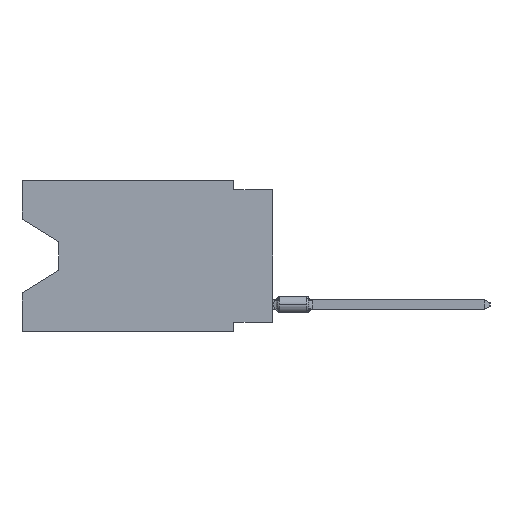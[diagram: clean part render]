
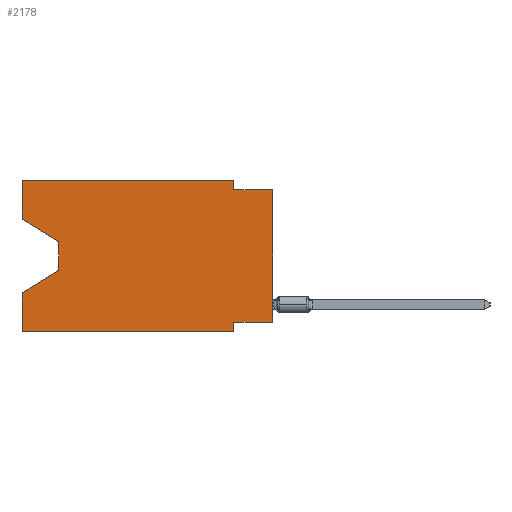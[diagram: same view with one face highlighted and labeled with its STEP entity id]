
A CAD part, left-side view. The second image highlights one B-rep face of the part: STEP entity #2178.
In plain terms, the highlighted planar face has unit normal (-1, 0, 0).
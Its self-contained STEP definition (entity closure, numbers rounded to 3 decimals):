
#2178 = ADVANCED_FACE ( 'NONE', ( #44456 ), #65878, .F. ) ;
#2504 = VERTEX_POINT ( 'NONE', #70240 ) ;
#3340 = ORIENTED_EDGE ( 'NONE', *, *, #38763, .F. ) ;
#3850 = VERTEX_POINT ( 'NONE', #56919 ) ;
#5890 = EDGE_CURVE ( 'NONE', #26819, #31688, #14589, .T. ) ;
#6187 = LINE ( 'NONE', #35373, #51066 ) ;
#7410 = VECTOR ( 'NONE', #53629, 1000. ) ;
#7866 = VECTOR ( 'NONE', #25039, 1000. ) ;
#8179 = EDGE_CURVE ( 'NONE', #27010, #69252, #20210, .T. ) ;
#8800 = DIRECTION ( 'NONE',  ( 0., 0., -1. ) ) ;
#9106 = ORIENTED_EDGE ( 'NONE', *, *, #55734, .T. ) ;
#9294 = CARTESIAN_POINT ( 'NONE',  ( 0., 2.54, 0. ) ) ;
#14589 = LINE ( 'NONE', #32712, #46270 ) ;
#15774 = EDGE_CURVE ( 'NONE', #3850, #2504, #6187, .T. ) ;
#16365 = CARTESIAN_POINT ( 'NONE',  ( 0., 0., -0.635 ) ) ;
#16790 = CARTESIAN_POINT ( 'NONE',  ( 0., 2.54, -0.635 ) ) ;
#17894 = VECTOR ( 'NONE', #57328, 1000. ) ;
#20210 = LINE ( 'NONE', #42770, #64176 ) ;
#23904 = EDGE_CURVE ( 'NONE', #27010, #28588, #71907, .T. ) ;
#24351 = ORIENTED_EDGE ( 'NONE', *, *, #54726, .F. ) ;
#24639 = ORIENTED_EDGE ( 'NONE', *, *, #45463, .F. ) ;
#25039 = DIRECTION ( 'NONE',  ( 0., 0., -1. ) ) ;
#26361 = DIRECTION ( 'NONE',  ( 0., 0., -1. ) ) ;
#26819 = VERTEX_POINT ( 'NONE', #43142 ) ;
#27010 = VERTEX_POINT ( 'NONE', #58485 ) ;
#27949 = DIRECTION ( 'NONE',  ( 0., 0., 1. ) ) ;
#28588 = VERTEX_POINT ( 'NONE', #60197 ) ;
#30990 = EDGE_CURVE ( 'NONE', #57679, #66327, #49240, .T. ) ;
#31113 = LINE ( 'NONE', #32211, #7410 ) ;
#31688 = VERTEX_POINT ( 'NONE', #71348 ) ;
#32211 = CARTESIAN_POINT ( 'NONE',  ( 0., 16.383, 0. ) ) ;
#32712 = CARTESIAN_POINT ( 'NONE',  ( 0., 16.383, -2.546 ) ) ;
#33764 = DIRECTION ( 'NONE',  ( 0., -1., 0. ) ) ;
#34282 = DIRECTION ( 'NONE',  ( 0., 0., 1. ) ) ;
#34669 = ORIENTED_EDGE ( 'NONE', *, *, #5890, .T. ) ;
#35373 = CARTESIAN_POINT ( 'NONE',  ( 0., 0., 0. ) ) ;
#37228 = DIRECTION ( 'NONE',  ( 0., -1., 0. ) ) ;
#37519 = ORIENTED_EDGE ( 'NONE', *, *, #69914, .F. ) ;
#38763 = EDGE_CURVE ( 'NONE', #63058, #69252, #70104, .T. ) ;
#39256 = LINE ( 'NONE', #56597, #60037 ) ;
#39663 = EDGE_CURVE ( 'NONE', #66327, #72418, #45112, .T. ) ;
#40683 = LINE ( 'NONE', #16365, #62429 ) ;
#40953 = ORIENTED_EDGE ( 'NONE', *, *, #30990, .F. ) ;
#41041 = DIRECTION ( 'NONE',  ( 0., 0., -1. ) ) ;
#41968 = CARTESIAN_POINT ( 'NONE',  ( 0., 2.54, -9.906 ) ) ;
#42770 = CARTESIAN_POINT ( 'NONE',  ( 0., 16.383, -9.906 ) ) ;
#43142 = CARTESIAN_POINT ( 'NONE',  ( 0., 16.383, -2.546 ) ) ;
#44456 = FACE_OUTER_BOUND ( 'NONE', #56795, .T. ) ;
#45112 = LINE ( 'NONE', #63183, #51645 ) ;
#45463 = EDGE_CURVE ( 'NONE', #26819, #57679, #31113, .T. ) ;
#45885 = VERTEX_POINT ( 'NONE', #64636 ) ;
#46270 = VECTOR ( 'NONE', #53761, 1000. ) ;
#47268 = VECTOR ( 'NONE', #71763, 1000. ) ;
#47351 = CARTESIAN_POINT ( 'NONE',  ( 0., 13.97, -5.893 ) ) ;
#48974 = CARTESIAN_POINT ( 'NONE',  ( 0., 2.54, -9.271 ) ) ;
#49240 = LINE ( 'NONE', #70301, #47268 ) ;
#49623 = DIRECTION ( 'NONE',  ( 1., 0., 0. ) ) ;
#50493 = ORIENTED_EDGE ( 'NONE', *, *, #39663, .F. ) ;
#50818 = CARTESIAN_POINT ( 'NONE',  ( 0., 16.383, 0. ) ) ;
#51066 = VECTOR ( 'NONE', #34282, 1000. ) ;
#51645 = VECTOR ( 'NONE', #41041, 1000. ) ;
#53629 = DIRECTION ( 'NONE',  ( 0., 0., 1. ) ) ;
#53761 = DIRECTION ( 'NONE',  ( 0., -0.855, -0.519 ) ) ;
#54726 = EDGE_CURVE ( 'NONE', #72418, #2504, #40683, .T. ) ;
#55734 = EDGE_CURVE ( 'NONE', #31688, #45885, #59415, .T. ) ;
#55890 = CARTESIAN_POINT ( 'NONE',  ( 0., 16.383, 0. ) ) ;
#56597 = CARTESIAN_POINT ( 'NONE',  ( 0., 0., -9.271 ) ) ;
#56795 = EDGE_LOOP ( 'NONE', ( #34669, #9106, #67326, #58137, #65698, #3340, #37519, #58535, #24351, #50493, #40953, #24639 ) ) ;
#56919 = CARTESIAN_POINT ( 'NONE',  ( 0., 0., -9.271 ) ) ;
#57328 = DIRECTION ( 'NONE',  ( 0., 0.855, -0.519 ) ) ;
#57679 = VERTEX_POINT ( 'NONE', #50818 ) ;
#58137 = ORIENTED_EDGE ( 'NONE', *, *, #23904, .F. ) ;
#58485 = CARTESIAN_POINT ( 'NONE',  ( 0., 16.383, -9.906 ) ) ;
#58535 = ORIENTED_EDGE ( 'NONE', *, *, #15774, .T. ) ;
#59415 = LINE ( 'NONE', #70140, #62529 ) ;
#60037 = VECTOR ( 'NONE', #62144, 1000. ) ;
#60197 = CARTESIAN_POINT ( 'NONE',  ( 0., 16.383, -7.36 ) ) ;
#62144 = DIRECTION ( 'NONE',  ( 0., 1., 0. ) ) ;
#62429 = VECTOR ( 'NONE', #33764, 1000. ) ;
#62529 = VECTOR ( 'NONE', #8800, 1000. ) ;
#63058 = VERTEX_POINT ( 'NONE', #48974 ) ;
#63183 = CARTESIAN_POINT ( 'NONE',  ( 0., 2.54, 0. ) ) ;
#63957 = LINE ( 'NONE', #47351, #17894 ) ;
#64176 = VECTOR ( 'NONE', #37228, 1000. ) ;
#64636 = CARTESIAN_POINT ( 'NONE',  ( 0., 13.97, -5.893 ) ) ;
#64780 = AXIS2_PLACEMENT_3D ( 'NONE', #55890, #49623, #26361 ) ;
#65698 = ORIENTED_EDGE ( 'NONE', *, *, #8179, .T. ) ;
#65878 = PLANE ( 'NONE',  #64780 ) ;
#66327 = VERTEX_POINT ( 'NONE', #9294 ) ;
#67089 = CARTESIAN_POINT ( 'NONE',  ( 0., 16.383, 0. ) ) ;
#67326 = ORIENTED_EDGE ( 'NONE', *, *, #72991, .T. ) ;
#68078 = VECTOR ( 'NONE', #27949, 1000. ) ;
#69252 = VERTEX_POINT ( 'NONE', #41968 ) ;
#69747 = CARTESIAN_POINT ( 'NONE',  ( 0., 2.54, -9.906 ) ) ;
#69914 = EDGE_CURVE ( 'NONE', #3850, #63058, #39256, .T. ) ;
#70104 = LINE ( 'NONE', #69747, #7866 ) ;
#70140 = CARTESIAN_POINT ( 'NONE',  ( 0., 13.97, -4.013 ) ) ;
#70240 = CARTESIAN_POINT ( 'NONE',  ( 0., 0., -0.635 ) ) ;
#70301 = CARTESIAN_POINT ( 'NONE',  ( 0., 16.383, 0. ) ) ;
#71348 = CARTESIAN_POINT ( 'NONE',  ( 0., 13.97, -4.013 ) ) ;
#71763 = DIRECTION ( 'NONE',  ( 0., -1., 0. ) ) ;
#71907 = LINE ( 'NONE', #67089, #68078 ) ;
#72418 = VERTEX_POINT ( 'NONE', #16790 ) ;
#72991 = EDGE_CURVE ( 'NONE', #45885, #28588, #63957, .T. ) ;
